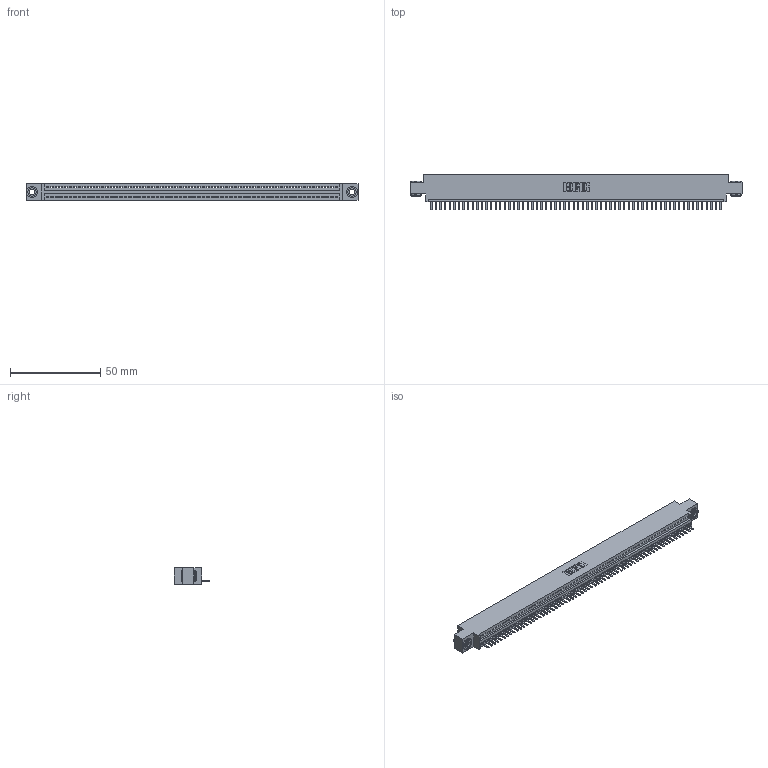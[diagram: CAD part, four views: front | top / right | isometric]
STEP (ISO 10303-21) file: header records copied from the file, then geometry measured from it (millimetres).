
FILE_DESCRIPTION (( 'STEP AP203' ), '1' );
FILE_NAME ('395-064-520-603.STEP', '2018-11-24T11:47:30', ( '' ), ( '' ), 'SwSTEP 2.0', 'SolidWorks 2016', '' );
FILE_SCHEMA (( 'CONFIG_CONTROL_DESIGN' ));
Length unit declared in the file: inch
Products named in the file (4): 345-250-002_345-250-002-102; 395-064-520-603; 345 Part_0.170 Offset - 0.156 Dia-TH; 345-292-001_345-293-120
Assembly tree (67 placements, depth 2):
  395-064-520-603
    345 Part_0.170 Offset - 0.156 Dia-TH
    345-292-001_345-293-120  x64
    345-250-002_345-250-002-102  x2
Bounding box: 183.77 x 19.68 x 9.4 mm (x, y, z)
Volume: 17356.7 mm3; surface area: 23103.2 mm2
Topology: 67 solids, 67 shells, 4136 faces, 12205 edges, 7962 vertices
Faces by surface type: plane 2782, cylinder 1346, cone 8
Entity records: 46102 total; most frequent: CARTESIAN_POINT 7975, ORIENTED_EDGE 7954, DIRECTION 6951, EDGE_CURVE 3977, VECTOR 3561, LINE 3561, VERTEX_POINT 2646, AXIS2_PLACEMENT_3D 1695
